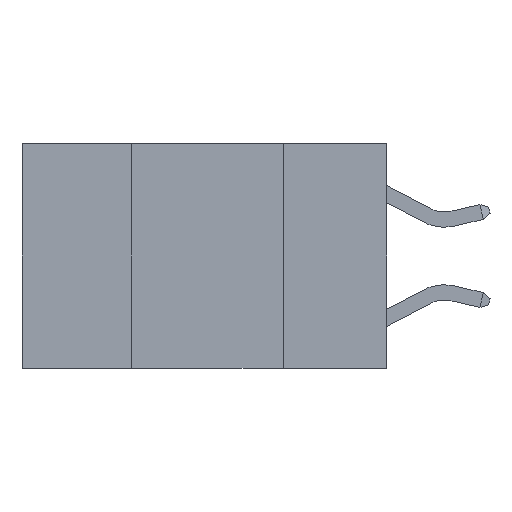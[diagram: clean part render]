
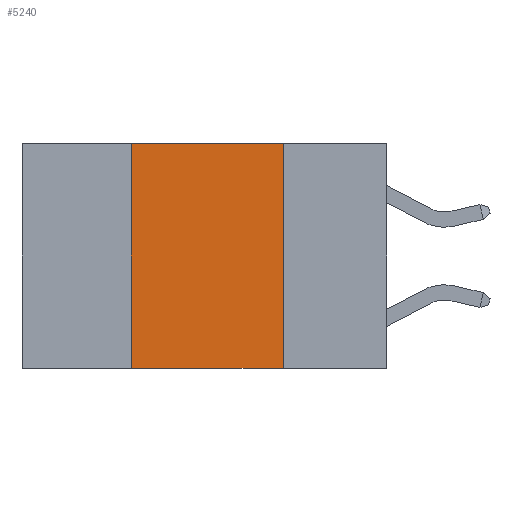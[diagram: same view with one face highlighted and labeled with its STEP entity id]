
A CAD part, left-side view. The second image highlights one B-rep face of the part: STEP entity #5240.
In plain terms, the highlighted planar face has unit normal (-1, 0, 0).
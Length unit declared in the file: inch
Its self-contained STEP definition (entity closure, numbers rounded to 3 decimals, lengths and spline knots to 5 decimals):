
#204 = EDGE_CURVE ( 'NONE', #6406, #11107, #13109, .T. ) ;
#821 = EDGE_CURVE ( 'NONE', #11107, #18356, #7546, .T. ) ;
#1482 = ORIENTED_EDGE ( 'NONE', *, *, #6864, .T. ) ;
#2447 = FACE_OUTER_BOUND ( 'NONE', #12555, .T. ) ;
#2979 = ORIENTED_EDGE ( 'NONE', *, *, #821, .F. ) ;
#3031 = VECTOR ( 'NONE', #15180, 39.37008 ) ;
#4173 = CARTESIAN_POINT ( 'NONE',  ( 0., 0.6, -0.37 ) ) ;
#4904 = DIRECTION ( 'NONE',  ( 0., 0., -1. ) ) ;
#5240 = ADVANCED_FACE ( 'NONE', ( #2447 ), #20079, .F. ) ;
#6406 = VERTEX_POINT ( 'NONE', #8790 ) ;
#6864 = EDGE_CURVE ( 'NONE', #12703, #18356, #15593, .T. ) ;
#6970 = CARTESIAN_POINT ( 'NONE',  ( 0., 0.6, 0. ) ) ;
#7546 = LINE ( 'NONE', #8045, #9126 ) ;
#8045 = CARTESIAN_POINT ( 'NONE',  ( 0., 0.17, 0. ) ) ;
#8219 = VECTOR ( 'NONE', #15383, 39.37008 ) ;
#8567 = DIRECTION ( 'NONE',  ( 1., 0., 0. ) ) ;
#8790 = CARTESIAN_POINT ( 'NONE',  ( 0., 0.42, 0. ) ) ;
#9126 = VECTOR ( 'NONE', #4904, 39.37008 ) ;
#9587 = DIRECTION ( 'NONE',  ( 0., -1., 0. ) ) ;
#10457 = VECTOR ( 'NONE', #9587, 39.37008 ) ;
#10538 = DIRECTION ( 'NONE',  ( 0., 0., -1. ) ) ;
#11107 = VERTEX_POINT ( 'NONE', #14126 ) ;
#11764 = LINE ( 'NONE', #16759, #3031 ) ;
#12063 = AXIS2_PLACEMENT_3D ( 'NONE', #6970, #8567, #10538 ) ;
#12555 = EDGE_LOOP ( 'NONE', ( #2979, #20164, #17401, #1482 ) ) ;
#12703 = VERTEX_POINT ( 'NONE', #14614 ) ;
#13109 = LINE ( 'NONE', #17283, #10457 ) ;
#13792 = EDGE_CURVE ( 'NONE', #12703, #6406, #11764, .T. ) ;
#13935 = CARTESIAN_POINT ( 'NONE',  ( 0., 0.17, -0.37 ) ) ;
#14126 = CARTESIAN_POINT ( 'NONE',  ( 0., 0.17, 0. ) ) ;
#14614 = CARTESIAN_POINT ( 'NONE',  ( 0., 0.42, -0.37 ) ) ;
#15180 = DIRECTION ( 'NONE',  ( 0., 0., 1. ) ) ;
#15383 = DIRECTION ( 'NONE',  ( 0., -1., 0. ) ) ;
#15593 = LINE ( 'NONE', #4173, #8219 ) ;
#16759 = CARTESIAN_POINT ( 'NONE',  ( 0., 0.42, 0. ) ) ;
#17283 = CARTESIAN_POINT ( 'NONE',  ( 0., 0.6, 0. ) ) ;
#17401 = ORIENTED_EDGE ( 'NONE', *, *, #13792, .F. ) ;
#18356 = VERTEX_POINT ( 'NONE', #13935 ) ;
#20079 = PLANE ( 'NONE',  #12063 ) ;
#20164 = ORIENTED_EDGE ( 'NONE', *, *, #204, .F. ) ;
